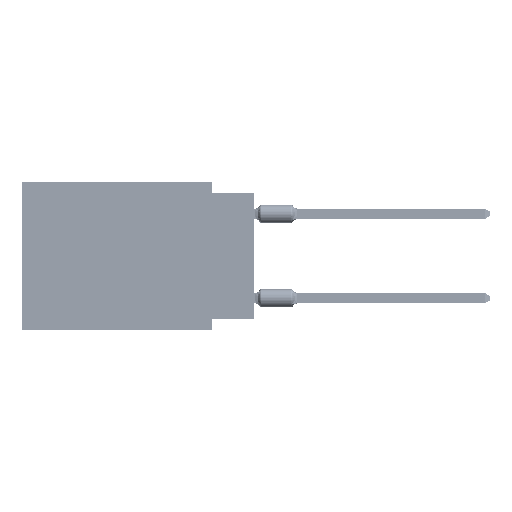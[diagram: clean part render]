
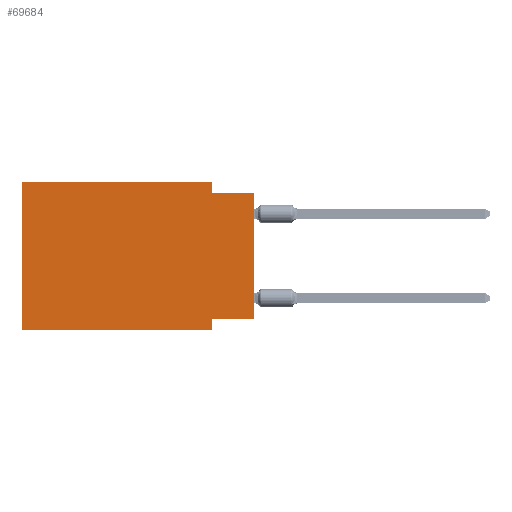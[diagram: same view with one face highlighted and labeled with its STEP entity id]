
A CAD part, left-side view. The second image highlights one B-rep face of the part: STEP entity #69684.
In plain terms, the highlighted planar face has unit normal (-1, 0, 0).
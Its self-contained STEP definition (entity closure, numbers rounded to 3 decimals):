
#635 = CARTESIAN_POINT ( 'NONE',  ( 0., 13.97, -8.89 ) ) ;
#1448 = EDGE_LOOP ( 'NONE', ( #38194, #24295, #7510, #51917, #56671, #51476, #54199, #22006 ) ) ;
#1969 = VECTOR ( 'NONE', #62571, 1000. ) ;
#2322 = LINE ( 'NONE', #66863, #14147 ) ;
#3358 = DIRECTION ( 'NONE',  ( 0., 0., -1. ) ) ;
#4638 = EDGE_CURVE ( 'NONE', #5676, #54175, #34870, .T. ) ;
#5676 = VERTEX_POINT ( 'NONE', #44997 ) ;
#5998 = CARTESIAN_POINT ( 'NONE',  ( 0., 2.54, -8.89 ) ) ;
#6019 = DIRECTION ( 'NONE',  ( 0., 1., 0. ) ) ;
#7510 = ORIENTED_EDGE ( 'NONE', *, *, #65387, .F. ) ;
#9935 = CARTESIAN_POINT ( 'NONE',  ( 0., 2.54, -8.89 ) ) ;
#10019 = CARTESIAN_POINT ( 'NONE',  ( 0., 0., 0. ) ) ;
#10555 = VERTEX_POINT ( 'NONE', #9935 ) ;
#12327 = VECTOR ( 'NONE', #61193, 1000. ) ;
#13322 = CARTESIAN_POINT ( 'NONE',  ( 0., 13.97, 0. ) ) ;
#14147 = VECTOR ( 'NONE', #72727, 1000. ) ;
#14783 = LINE ( 'NONE', #67653, #1969 ) ;
#14920 = VECTOR ( 'NONE', #63849, 1000. ) ;
#15033 = CARTESIAN_POINT ( 'NONE',  ( 0., 13.97, 0. ) ) ;
#15247 = LINE ( 'NONE', #45917, #57491 ) ;
#16324 = CARTESIAN_POINT ( 'NONE',  ( 0., 2.54, -0.635 ) ) ;
#17315 = VECTOR ( 'NONE', #76856, 1000. ) ;
#17355 = VERTEX_POINT ( 'NONE', #13322 ) ;
#17960 = CARTESIAN_POINT ( 'NONE',  ( 0., 2.54, 0. ) ) ;
#18457 = CARTESIAN_POINT ( 'NONE',  ( 0., 0., -8.255 ) ) ;
#19799 = VECTOR ( 'NONE', #52653, 1000. ) ;
#22006 = ORIENTED_EDGE ( 'NONE', *, *, #68295, .F. ) ;
#24295 = ORIENTED_EDGE ( 'NONE', *, *, #48656, .F. ) ;
#26015 = EDGE_CURVE ( 'NONE', #17355, #75611, #2322, .T. ) ;
#29327 = LINE ( 'NONE', #5998, #19799 ) ;
#30847 = VERTEX_POINT ( 'NONE', #43833 ) ;
#34870 = LINE ( 'NONE', #10019, #17315 ) ;
#38194 = ORIENTED_EDGE ( 'NONE', *, *, #4638, .T. ) ;
#39019 = CARTESIAN_POINT ( 'NONE',  ( 0., 0., -0.635 ) ) ;
#40502 = EDGE_CURVE ( 'NONE', #70898, #17355, #15247, .T. ) ;
#43833 = CARTESIAN_POINT ( 'NONE',  ( 0., 2.54, -8.255 ) ) ;
#44573 = DIRECTION ( 'NONE',  ( 1., 0., 0. ) ) ;
#44819 = VECTOR ( 'NONE', #6019, 1000. ) ;
#44997 = CARTESIAN_POINT ( 'NONE',  ( 0., 0., -8.255 ) ) ;
#45917 = CARTESIAN_POINT ( 'NONE',  ( 0., 13.97, 0. ) ) ;
#48656 = EDGE_CURVE ( 'NONE', #58401, #54175, #50290, .T. ) ;
#50290 = LINE ( 'NONE', #39019, #12327 ) ;
#51476 = ORIENTED_EDGE ( 'NONE', *, *, #75230, .T. ) ;
#51754 = DIRECTION ( 'NONE',  ( 0., 0., 1. ) ) ;
#51917 = ORIENTED_EDGE ( 'NONE', *, *, #26015, .F. ) ;
#52562 = LINE ( 'NONE', #17960, #14920 ) ;
#52653 = DIRECTION ( 'NONE',  ( 0., 0., -1. ) ) ;
#54175 = VERTEX_POINT ( 'NONE', #62897 ) ;
#54199 = ORIENTED_EDGE ( 'NONE', *, *, #65007, .F. ) ;
#56606 = FACE_OUTER_BOUND ( 'NONE', #1448, .T. ) ;
#56671 = ORIENTED_EDGE ( 'NONE', *, *, #40502, .F. ) ;
#57491 = VECTOR ( 'NONE', #51754, 1000. ) ;
#58401 = VERTEX_POINT ( 'NONE', #16324 ) ;
#61193 = DIRECTION ( 'NONE',  ( 0., -1., 0. ) ) ;
#62571 = DIRECTION ( 'NONE',  ( 0., -1., 0. ) ) ;
#62897 = CARTESIAN_POINT ( 'NONE',  ( 0., 0., -0.635 ) ) ;
#63593 = PLANE ( 'NONE',  #68554 ) ;
#63849 = DIRECTION ( 'NONE',  ( 0., 0., -1. ) ) ;
#65007 = EDGE_CURVE ( 'NONE', #30847, #10555, #29327, .T. ) ;
#65387 = EDGE_CURVE ( 'NONE', #75611, #58401, #52562, .T. ) ;
#66863 = CARTESIAN_POINT ( 'NONE',  ( 0., 13.97, 0. ) ) ;
#67653 = CARTESIAN_POINT ( 'NONE',  ( 0., 13.97, -8.89 ) ) ;
#68295 = EDGE_CURVE ( 'NONE', #5676, #30847, #71725, .T. ) ;
#68554 = AXIS2_PLACEMENT_3D ( 'NONE', #15033, #44573, #3358 ) ;
#68688 = CARTESIAN_POINT ( 'NONE',  ( 0., 2.54, 0. ) ) ;
#69684 = ADVANCED_FACE ( 'NONE', ( #56606 ), #63593, .F. ) ;
#70898 = VERTEX_POINT ( 'NONE', #635 ) ;
#71725 = LINE ( 'NONE', #18457, #44819 ) ;
#72727 = DIRECTION ( 'NONE',  ( 0., -1., 0. ) ) ;
#75230 = EDGE_CURVE ( 'NONE', #70898, #10555, #14783, .T. ) ;
#75611 = VERTEX_POINT ( 'NONE', #68688 ) ;
#76856 = DIRECTION ( 'NONE',  ( 0., 0., 1. ) ) ;
